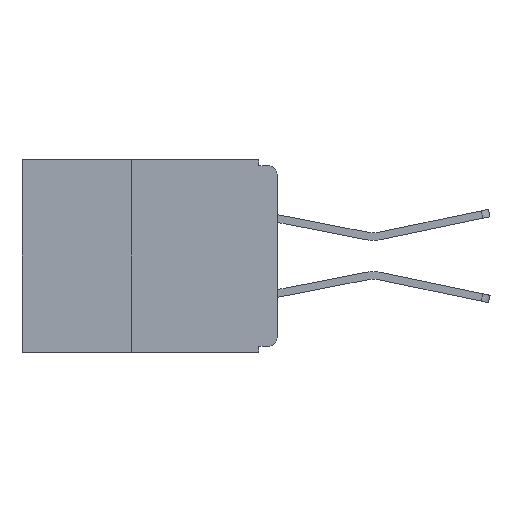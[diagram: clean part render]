
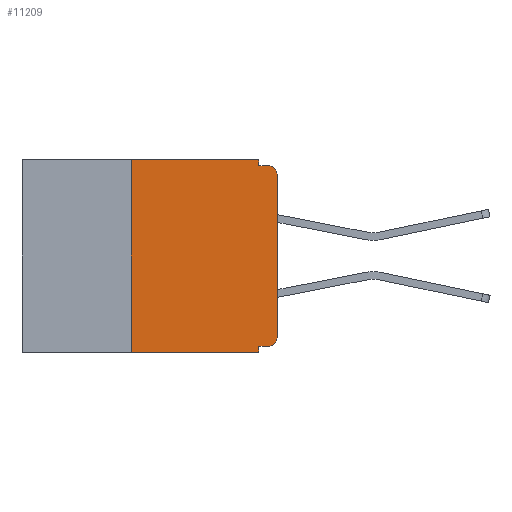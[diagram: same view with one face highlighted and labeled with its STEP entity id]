
A CAD part, left-side view. The second image highlights one B-rep face of the part: STEP entity #11209.
In plain terms, the highlighted planar face has unit normal (-1, 0, 0).
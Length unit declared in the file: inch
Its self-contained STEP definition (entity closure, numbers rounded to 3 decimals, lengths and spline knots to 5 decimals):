
#176 = DIRECTION ( 'NONE',  ( 0., 0., 1. ) ) ;
#275 = CARTESIAN_POINT ( 'NONE',  ( 0., 0.015, -0.32 ) ) ;
#301 = PLANE ( 'NONE',  #4514 ) ;
#352 = CARTESIAN_POINT ( 'NONE',  ( 0., 0., 0. ) ) ;
#886 = CARTESIAN_POINT ( 'NONE',  ( 0., 0.031, -0.33 ) ) ;
#962 = CARTESIAN_POINT ( 'NONE',  ( 0., 0.437, 0. ) ) ;
#1400 = LINE ( 'NONE', #7823, #7037 ) ;
#1402 = CARTESIAN_POINT ( 'NONE',  ( 0., 0.25, -0.33 ) ) ;
#1957 = VERTEX_POINT ( 'NONE', #5749 ) ;
#2262 = VECTOR ( 'NONE', #4840, 39.37008 ) ;
#2818 = CARTESIAN_POINT ( 'NONE',  ( 0., 0.25, -0.33 ) ) ;
#2894 = EDGE_CURVE ( 'NONE', #13047, #1957, #8665, .T. ) ;
#3009 = ORIENTED_EDGE ( 'NONE', *, *, #5709, .T. ) ;
#3086 = EDGE_CURVE ( 'NONE', #1957, #10879, #8837, .T. ) ;
#3543 = VERTEX_POINT ( 'NONE', #12234 ) ;
#3716 = VERTEX_POINT ( 'NONE', #9996 ) ;
#3790 = DIRECTION ( 'NONE',  ( 0., 0., -1. ) ) ;
#3794 = DIRECTION ( 'NONE',  ( -1., 0., 0. ) ) ;
#3812 = CARTESIAN_POINT ( 'NONE',  ( 0., 0.015, -0.025 ) ) ;
#3858 = VERTEX_POINT ( 'NONE', #8403 ) ;
#3927 = EDGE_CURVE ( 'NONE', #12841, #7845, #7593, .T. ) ;
#4120 = CARTESIAN_POINT ( 'NONE',  ( 0., 0.015, -0.305 ) ) ;
#4254 = VERTEX_POINT ( 'NONE', #2818 ) ;
#4376 = DIRECTION ( 'NONE',  ( 0., 0., -1. ) ) ;
#4407 = DIRECTION ( 'NONE',  ( -1., 0., 0. ) ) ;
#4514 = AXIS2_PLACEMENT_3D ( 'NONE', #11503, #13715, #7108 ) ;
#4838 = ORIENTED_EDGE ( 'NONE', *, *, #5931, .T. ) ;
#4840 = DIRECTION ( 'NONE',  ( 0., 0., 1. ) ) ;
#5028 = ORIENTED_EDGE ( 'NONE', *, *, #10853, .F. ) ;
#5106 = VECTOR ( 'NONE', #5356, 39.37008 ) ;
#5356 = DIRECTION ( 'NONE',  ( 0., -1., 0. ) ) ;
#5377 = CARTESIAN_POINT ( 'NONE',  ( 0., 0.437, -0.33 ) ) ;
#5691 = LINE ( 'NONE', #8578, #13481 ) ;
#5709 = EDGE_CURVE ( 'NONE', #4254, #11521, #10672, .T. ) ;
#5749 = CARTESIAN_POINT ( 'NONE',  ( 0., 0., -0.305 ) ) ;
#5868 = AXIS2_PLACEMENT_3D ( 'NONE', #3812, #3794, #3790 ) ;
#5869 = VECTOR ( 'NONE', #176, 39.37008 ) ;
#5931 = EDGE_CURVE ( 'NONE', #10879, #3543, #13427, .T. ) ;
#6246 = DIRECTION ( 'NONE',  ( 0., -1., 0. ) ) ;
#6875 = VECTOR ( 'NONE', #11627, 39.37008 ) ;
#7037 = VECTOR ( 'NONE', #10058, 39.37008 ) ;
#7108 = DIRECTION ( 'NONE',  ( 0., 0., -1. ) ) ;
#7128 = CARTESIAN_POINT ( 'NONE',  ( 0., 0.031, 0. ) ) ;
#7245 = VECTOR ( 'NONE', #7445, 39.37008 ) ;
#7445 = DIRECTION ( 'NONE',  ( 0., 0., -1. ) ) ;
#7513 = CARTESIAN_POINT ( 'NONE',  ( 0., 0., -0.025 ) ) ;
#7593 = LINE ( 'NONE', #7128, #7245 ) ;
#7823 = CARTESIAN_POINT ( 'NONE',  ( 0., 0.031, -0.33 ) ) ;
#7845 = VERTEX_POINT ( 'NONE', #11308 ) ;
#7918 = ORIENTED_EDGE ( 'NONE', *, *, #12594, .F. ) ;
#7961 = EDGE_CURVE ( 'NONE', #4254, #3858, #14438, .T. ) ;
#8403 = CARTESIAN_POINT ( 'NONE',  ( 0., 0.25, 0. ) ) ;
#8578 = CARTESIAN_POINT ( 'NONE',  ( 0., 0., -0.01 ) ) ;
#8665 = CIRCLE ( 'NONE', #14080, 0.015 ) ;
#8837 = LINE ( 'NONE', #352, #5869 ) ;
#9010 = ORIENTED_EDGE ( 'NONE', *, *, #3086, .T. ) ;
#9410 = ORIENTED_EDGE ( 'NONE', *, *, #13408, .F. ) ;
#9601 = ORIENTED_EDGE ( 'NONE', *, *, #7961, .F. ) ;
#9996 = CARTESIAN_POINT ( 'NONE',  ( 0., 0.031, -0.32 ) ) ;
#10058 = DIRECTION ( 'NONE',  ( 0., 0., -1. ) ) ;
#10508 = LINE ( 'NONE', #962, #13093 ) ;
#10672 = LINE ( 'NONE', #5377, #5106 ) ;
#10779 = ORIENTED_EDGE ( 'NONE', *, *, #2894, .T. ) ;
#10853 = EDGE_CURVE ( 'NONE', #7845, #3543, #5691, .T. ) ;
#10879 = VERTEX_POINT ( 'NONE', #7513 ) ;
#11209 = ADVANCED_FACE ( 'NONE', ( #11232 ), #301, .F. ) ;
#11232 = FACE_OUTER_BOUND ( 'NONE', #14013, .T. ) ;
#11308 = CARTESIAN_POINT ( 'NONE',  ( 0., 0.031, -0.01 ) ) ;
#11503 = CARTESIAN_POINT ( 'NONE',  ( 0., 0.437, 0. ) ) ;
#11521 = VERTEX_POINT ( 'NONE', #886 ) ;
#11582 = CARTESIAN_POINT ( 'NONE',  ( 0., 0., -0.32 ) ) ;
#11627 = DIRECTION ( 'NONE',  ( 0., 1., 0. ) ) ;
#12234 = CARTESIAN_POINT ( 'NONE',  ( 0., 0.015, -0.01 ) ) ;
#12594 = EDGE_CURVE ( 'NONE', #13047, #3716, #12732, .T. ) ;
#12732 = LINE ( 'NONE', #11582, #6875 ) ;
#12841 = VERTEX_POINT ( 'NONE', #14226 ) ;
#13047 = VERTEX_POINT ( 'NONE', #275 ) ;
#13093 = VECTOR ( 'NONE', #13255, 39.37008 ) ;
#13255 = DIRECTION ( 'NONE',  ( 0., -1., 0. ) ) ;
#13408 = EDGE_CURVE ( 'NONE', #3858, #12841, #10508, .T. ) ;
#13412 = ORIENTED_EDGE ( 'NONE', *, *, #14136, .F. ) ;
#13427 = CIRCLE ( 'NONE', #5868, 0.015 ) ;
#13481 = VECTOR ( 'NONE', #6246, 39.37008 ) ;
#13529 = ORIENTED_EDGE ( 'NONE', *, *, #3927, .F. ) ;
#13715 = DIRECTION ( 'NONE',  ( 1., 0., 0. ) ) ;
#14013 = EDGE_LOOP ( 'NONE', ( #9010, #4838, #5028, #13529, #9410, #9601, #3009, #13412, #7918, #10779 ) ) ;
#14080 = AXIS2_PLACEMENT_3D ( 'NONE', #4120, #4407, #4376 ) ;
#14136 = EDGE_CURVE ( 'NONE', #3716, #11521, #1400, .T. ) ;
#14226 = CARTESIAN_POINT ( 'NONE',  ( 0., 0.031, 0. ) ) ;
#14438 = LINE ( 'NONE', #1402, #2262 ) ;
